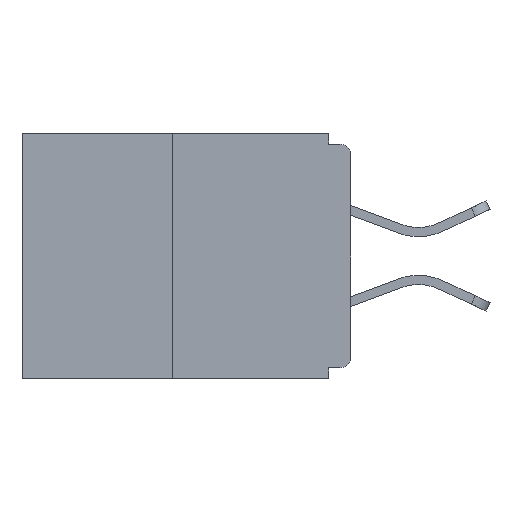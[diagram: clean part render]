
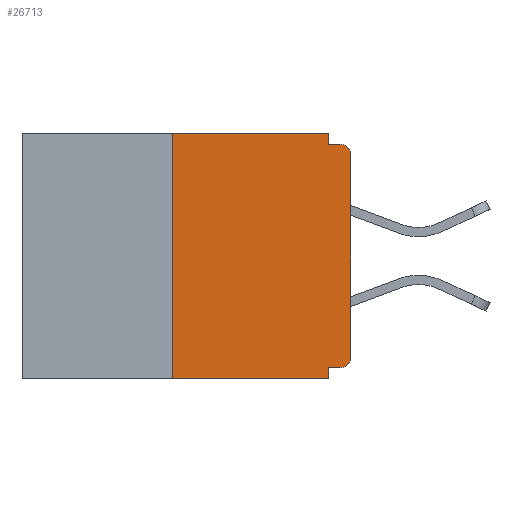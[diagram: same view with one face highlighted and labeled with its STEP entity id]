
A CAD part, left-side view. The second image highlights one B-rep face of the part: STEP entity #26713.
In plain terms, the highlighted planar face has unit normal (-1, 0, 0).
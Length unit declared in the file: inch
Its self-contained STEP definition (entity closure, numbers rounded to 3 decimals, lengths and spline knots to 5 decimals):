
#228 = EDGE_CURVE ( 'NONE', #4313, #15305, #12415, .T. ) ;
#771 = ORIENTED_EDGE ( 'NONE', *, *, #18160, .F. ) ;
#949 = CARTESIAN_POINT ( 'NONE',  ( 0., 0.25, -0.343 ) ) ;
#1397 = CIRCLE ( 'NONE', #12242, 0.015 ) ;
#1436 = VECTOR ( 'NONE', #11021, 39.37008 ) ;
#1525 = VECTOR ( 'NONE', #9583, 39.37008 ) ;
#1539 = CARTESIAN_POINT ( 'NONE',  ( 0., 0., 0. ) ) ;
#1826 = AXIS2_PLACEMENT_3D ( 'NONE', #8479, #6380, #14991 ) ;
#2975 = CARTESIAN_POINT ( 'NONE',  ( 0., 0.46, -0.343 ) ) ;
#3252 = VERTEX_POINT ( 'NONE', #949 ) ;
#3988 = VERTEX_POINT ( 'NONE', #12442 ) ;
#4313 = VERTEX_POINT ( 'NONE', #18577 ) ;
#4345 = CARTESIAN_POINT ( 'NONE',  ( 0., 0.015, -0.015 ) ) ;
#5241 = EDGE_CURVE ( 'NONE', #20735, #3988, #24713, .T. ) ;
#5573 = ORIENTED_EDGE ( 'NONE', *, *, #25811, .T. ) ;
#6380 = DIRECTION ( 'NONE',  ( -1., 0., 0. ) ) ;
#6503 = CARTESIAN_POINT ( 'NONE',  ( 0., 0.031, 0. ) ) ;
#6533 = VECTOR ( 'NONE', #16501, 39.37008 ) ;
#6730 = EDGE_CURVE ( 'NONE', #27427, #27367, #27220, .T. ) ;
#6964 = CARTESIAN_POINT ( 'NONE',  ( 0., 0.015, -0.03 ) ) ;
#7121 = ORIENTED_EDGE ( 'NONE', *, *, #6730, .F. ) ;
#7383 = ORIENTED_EDGE ( 'NONE', *, *, #27620, .F. ) ;
#7884 = CARTESIAN_POINT ( 'NONE',  ( 0., 0.46, 0. ) ) ;
#8479 = CARTESIAN_POINT ( 'NONE',  ( 0., 0.015, -0.313 ) ) ;
#9583 = DIRECTION ( 'NONE',  ( 0., -1., 0. ) ) ;
#10364 = ORIENTED_EDGE ( 'NONE', *, *, #10651, .T. ) ;
#10416 = VERTEX_POINT ( 'NONE', #13199 ) ;
#10472 = LINE ( 'NONE', #6503, #1436 ) ;
#10651 = EDGE_CURVE ( 'NONE', #20735, #4313, #16244, .T. ) ;
#10752 = CARTESIAN_POINT ( 'NONE',  ( 0., 0.015, -0.328 ) ) ;
#11021 = DIRECTION ( 'NONE',  ( 0., 0., -1. ) ) ;
#12137 = LINE ( 'NONE', #18339, #1525 ) ;
#12242 = AXIS2_PLACEMENT_3D ( 'NONE', #6964, #17545, #26032 ) ;
#12415 = LINE ( 'NONE', #1539, #18724 ) ;
#12442 = CARTESIAN_POINT ( 'NONE',  ( 0., 0.031, -0.328 ) ) ;
#12625 = ORIENTED_EDGE ( 'NONE', *, *, #228, .T. ) ;
#12764 = EDGE_CURVE ( 'NONE', #15305, #18768, #1397, .T. ) ;
#12877 = LINE ( 'NONE', #25568, #16712 ) ;
#13199 = CARTESIAN_POINT ( 'NONE',  ( 0., 0.031, -0.343 ) ) ;
#14168 = VERTEX_POINT ( 'NONE', #27352 ) ;
#14290 = CARTESIAN_POINT ( 'NONE',  ( 0., 0., -0.328 ) ) ;
#14296 = DIRECTION ( 'NONE',  ( 0., 0., -1. ) ) ;
#14564 = DIRECTION ( 'NONE',  ( 0., 0., 1. ) ) ;
#14568 = PLANE ( 'NONE',  #15851 ) ;
#14991 = DIRECTION ( 'NONE',  ( 0., 0., -1. ) ) ;
#15264 = EDGE_CURVE ( 'NONE', #14168, #18768, #12137, .T. ) ;
#15305 = VERTEX_POINT ( 'NONE', #25114 ) ;
#15674 = LINE ( 'NONE', #2975, #21667 ) ;
#15851 = AXIS2_PLACEMENT_3D ( 'NONE', #23166, #18933, #14296 ) ;
#16244 = CIRCLE ( 'NONE', #1826, 0.015 ) ;
#16443 = LINE ( 'NONE', #22781, #24910 ) ;
#16501 = DIRECTION ( 'NONE',  ( 0., -1., 0. ) ) ;
#16712 = VECTOR ( 'NONE', #14564, 39.37008 ) ;
#17545 = DIRECTION ( 'NONE',  ( -1., 0., 0. ) ) ;
#18160 = EDGE_CURVE ( 'NONE', #3252, #27427, #12877, .T. ) ;
#18339 = CARTESIAN_POINT ( 'NONE',  ( 0., 0., -0.015 ) ) ;
#18577 = CARTESIAN_POINT ( 'NONE',  ( 0., 0., -0.313 ) ) ;
#18724 = VECTOR ( 'NONE', #27353, 39.37008 ) ;
#18768 = VERTEX_POINT ( 'NONE', #4345 ) ;
#18933 = DIRECTION ( 'NONE',  ( 1., 0., 0. ) ) ;
#19046 = CARTESIAN_POINT ( 'NONE',  ( 0., 0.25, 0. ) ) ;
#20735 = VERTEX_POINT ( 'NONE', #10752 ) ;
#21667 = VECTOR ( 'NONE', #26536, 39.37008 ) ;
#22121 = ORIENTED_EDGE ( 'NONE', *, *, #12764, .T. ) ;
#22537 = ORIENTED_EDGE ( 'NONE', *, *, #15264, .F. ) ;
#22781 = CARTESIAN_POINT ( 'NONE',  ( 0., 0.031, -0.343 ) ) ;
#23166 = CARTESIAN_POINT ( 'NONE',  ( 0., 0.46, 0. ) ) ;
#23186 = EDGE_LOOP ( 'NONE', ( #7121, #771, #5573, #7383, #25125, #10364, #12625, #22121, #22537, #24774 ) ) ;
#23274 = CARTESIAN_POINT ( 'NONE',  ( 0., 0.031, 0. ) ) ;
#24713 = LINE ( 'NONE', #14290, #26164 ) ;
#24774 = ORIENTED_EDGE ( 'NONE', *, *, #26942, .F. ) ;
#24866 = FACE_OUTER_BOUND ( 'NONE', #23186, .T. ) ;
#24910 = VECTOR ( 'NONE', #27425, 39.37008 ) ;
#25114 = CARTESIAN_POINT ( 'NONE',  ( 0., 0., -0.03 ) ) ;
#25125 = ORIENTED_EDGE ( 'NONE', *, *, #5241, .F. ) ;
#25568 = CARTESIAN_POINT ( 'NONE',  ( 0., 0.25, 0. ) ) ;
#25811 = EDGE_CURVE ( 'NONE', #3252, #10416, #15674, .T. ) ;
#26032 = DIRECTION ( 'NONE',  ( 0., 0., -1. ) ) ;
#26164 = VECTOR ( 'NONE', #26966, 39.37008 ) ;
#26536 = DIRECTION ( 'NONE',  ( 0., -1., 0. ) ) ;
#26713 = ADVANCED_FACE ( 'NONE', ( #24866 ), #14568, .F. ) ;
#26942 = EDGE_CURVE ( 'NONE', #27367, #14168, #10472, .T. ) ;
#26966 = DIRECTION ( 'NONE',  ( 0., 1., 0. ) ) ;
#27220 = LINE ( 'NONE', #7884, #6533 ) ;
#27352 = CARTESIAN_POINT ( 'NONE',  ( 0., 0.031, -0.015 ) ) ;
#27353 = DIRECTION ( 'NONE',  ( 0., 0., 1. ) ) ;
#27367 = VERTEX_POINT ( 'NONE', #23274 ) ;
#27425 = DIRECTION ( 'NONE',  ( 0., 0., -1. ) ) ;
#27427 = VERTEX_POINT ( 'NONE', #19046 ) ;
#27620 = EDGE_CURVE ( 'NONE', #3988, #10416, #16443, .T. ) ;
